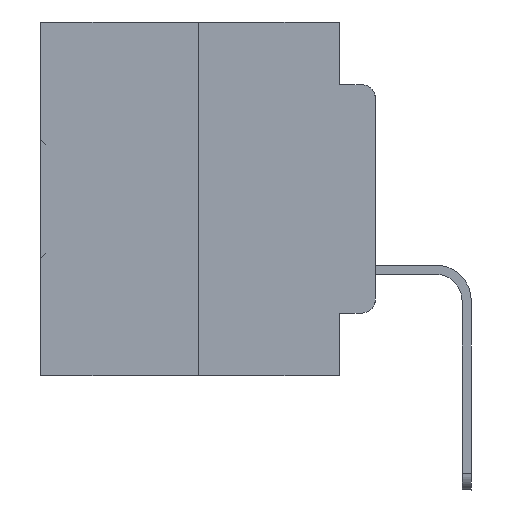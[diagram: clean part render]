
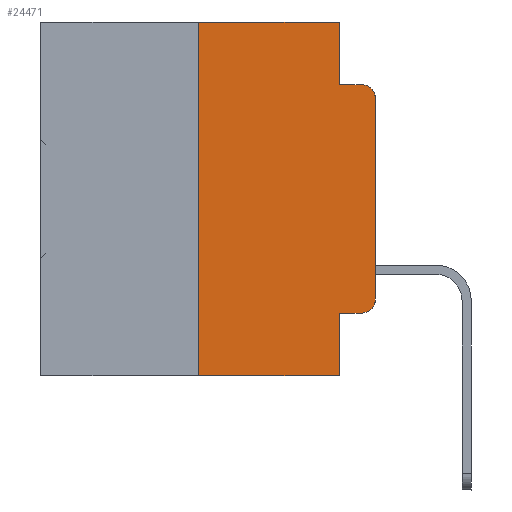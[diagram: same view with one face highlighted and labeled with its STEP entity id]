
A CAD part, left-side view. The second image highlights one B-rep face of the part: STEP entity #24471.
In plain terms, the highlighted planar face has unit normal (-1, 0, 0).
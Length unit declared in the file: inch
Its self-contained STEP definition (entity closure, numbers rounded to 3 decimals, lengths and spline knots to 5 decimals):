
#53 = EDGE_CURVE ( 'NONE', #14800, #1571, #8397, .T. ) ;
#319 = EDGE_CURVE ( 'NONE', #7575, #12504, #31278, .T. ) ;
#398 = CARTESIAN_POINT ( 'NONE',  ( 0., 0.473, 0. ) ) ;
#1571 = VERTEX_POINT ( 'NONE', #5385 ) ;
#2009 = VECTOR ( 'NONE', #22355, 39.37008 ) ;
#2048 = DIRECTION ( 'NONE',  ( 0., 0., 1. ) ) ;
#3149 = CARTESIAN_POINT ( 'NONE',  ( 0., 0.051, -0.0885 ) ) ;
#3265 = DIRECTION ( 'NONE',  ( 0., -1., 0. ) ) ;
#4979 = CARTESIAN_POINT ( 'NONE',  ( 0., 0.25, 0. ) ) ;
#5385 = CARTESIAN_POINT ( 'NONE',  ( 0., 0.02, -0.4115 ) ) ;
#5446 = DIRECTION ( 'NONE',  ( 0., 0., -1. ) ) ;
#5786 = CARTESIAN_POINT ( 'NONE',  ( 0., 0.473, 0. ) ) ;
#5818 = CIRCLE ( 'NONE', #23618, 0.02 ) ;
#5857 = CARTESIAN_POINT ( 'NONE',  ( 0., 0.051, 0. ) ) ;
#6010 = DIRECTION ( 'NONE',  ( 0., -1., 0. ) ) ;
#6371 = LINE ( 'NONE', #5786, #22662 ) ;
#6525 = EDGE_CURVE ( 'NONE', #14800, #15217, #8008, .T. ) ;
#6798 = CARTESIAN_POINT ( 'NONE',  ( 0., 0.02, -0.1085 ) ) ;
#6821 = CARTESIAN_POINT ( 'NONE',  ( 0., 0.051, -0.0885 ) ) ;
#6866 = EDGE_CURVE ( 'NONE', #22775, #15217, #16119, .T. ) ;
#7342 = EDGE_CURVE ( 'NONE', #12727, #27917, #7940, .T. ) ;
#7575 = VERTEX_POINT ( 'NONE', #9803 ) ;
#7852 = FACE_OUTER_BOUND ( 'NONE', #10377, .T. ) ;
#7940 = LINE ( 'NONE', #5857, #22614 ) ;
#8008 = LINE ( 'NONE', #22878, #21020 ) ;
#8397 = LINE ( 'NONE', #16643, #8834 ) ;
#8607 = VECTOR ( 'NONE', #32859, 39.37008 ) ;
#8613 = LINE ( 'NONE', #12088, #2009 ) ;
#8834 = VECTOR ( 'NONE', #20161, 39.37008 ) ;
#8839 = ORIENTED_EDGE ( 'NONE', *, *, #27946, .F. ) ;
#8915 = EDGE_CURVE ( 'NONE', #12504, #33897, #26978, .T. ) ;
#9507 = DIRECTION ( 'NONE',  ( 0., 0., -1. ) ) ;
#9710 = CARTESIAN_POINT ( 'NONE',  ( 0., 0.25, -0.5 ) ) ;
#9803 = CARTESIAN_POINT ( 'NONE',  ( 0., 0., -0.3915 ) ) ;
#10377 = EDGE_LOOP ( 'NONE', ( #31611, #15727, #30121, #11765, #8839, #25581, #11801, #24470, #13505, #22154 ) ) ;
#11185 = CARTESIAN_POINT ( 'NONE',  ( 0., 0.051, -0.4115 ) ) ;
#11765 = ORIENTED_EDGE ( 'NONE', *, *, #7342, .F. ) ;
#11801 = ORIENTED_EDGE ( 'NONE', *, *, #6866, .T. ) ;
#11934 = CARTESIAN_POINT ( 'NONE',  ( 0., 0.051, -0.5 ) ) ;
#11978 = AXIS2_PLACEMENT_3D ( 'NONE', #6798, #25012, #9507 ) ;
#12088 = CARTESIAN_POINT ( 'NONE',  ( 0., 0.25, 0. ) ) ;
#12365 = EDGE_CURVE ( 'NONE', #1571, #7575, #5818, .T. ) ;
#12504 = VERTEX_POINT ( 'NONE', #21328 ) ;
#12727 = VERTEX_POINT ( 'NONE', #30063 ) ;
#13059 = PLANE ( 'NONE',  #21486 ) ;
#13505 = ORIENTED_EDGE ( 'NONE', *, *, #53, .T. ) ;
#14800 = VERTEX_POINT ( 'NONE', #11185 ) ;
#14801 = DIRECTION ( 'NONE',  ( 0., 0., -1. ) ) ;
#15217 = VERTEX_POINT ( 'NONE', #11934 ) ;
#15727 = ORIENTED_EDGE ( 'NONE', *, *, #8915, .T. ) ;
#16119 = LINE ( 'NONE', #16453, #29641 ) ;
#16299 = DIRECTION ( 'NONE',  ( 0., 0., -1. ) ) ;
#16453 = CARTESIAN_POINT ( 'NONE',  ( 0., 0.473, -0.5 ) ) ;
#16643 = CARTESIAN_POINT ( 'NONE',  ( 0., 0.051, -0.4115 ) ) ;
#18079 = EDGE_CURVE ( 'NONE', #27917, #33897, #27358, .T. ) ;
#18781 = EDGE_CURVE ( 'NONE', #22775, #27675, #8613, .T. ) ;
#19354 = VECTOR ( 'NONE', #2048, 39.37008 ) ;
#20034 = CARTESIAN_POINT ( 'NONE',  ( 0., 0., 0. ) ) ;
#20161 = DIRECTION ( 'NONE',  ( 0., -1., 0. ) ) ;
#20626 = DIRECTION ( 'NONE',  ( -1., 0., 0. ) ) ;
#21020 = VECTOR ( 'NONE', #14801, 39.37008 ) ;
#21328 = CARTESIAN_POINT ( 'NONE',  ( 0., 0., -0.1085 ) ) ;
#21486 = AXIS2_PLACEMENT_3D ( 'NONE', #398, #29082, #5446 ) ;
#22154 = ORIENTED_EDGE ( 'NONE', *, *, #12365, .T. ) ;
#22355 = DIRECTION ( 'NONE',  ( 0., 0., 1. ) ) ;
#22614 = VECTOR ( 'NONE', #16299, 39.37008 ) ;
#22662 = VECTOR ( 'NONE', #3265, 39.37008 ) ;
#22775 = VERTEX_POINT ( 'NONE', #9710 ) ;
#22878 = CARTESIAN_POINT ( 'NONE',  ( 0., 0.051, 0. ) ) ;
#23381 = DIRECTION ( 'NONE',  ( 0., 0., -1. ) ) ;
#23618 = AXIS2_PLACEMENT_3D ( 'NONE', #26012, #20626, #23381 ) ;
#24470 = ORIENTED_EDGE ( 'NONE', *, *, #6525, .F. ) ;
#24471 = ADVANCED_FACE ( 'NONE', ( #7852 ), #13059, .F. ) ;
#25012 = DIRECTION ( 'NONE',  ( -1., 0., 0. ) ) ;
#25581 = ORIENTED_EDGE ( 'NONE', *, *, #18781, .F. ) ;
#26012 = CARTESIAN_POINT ( 'NONE',  ( 0., 0.02, -0.3915 ) ) ;
#26978 = CIRCLE ( 'NONE', #11978, 0.02 ) ;
#27358 = LINE ( 'NONE', #6821, #8607 ) ;
#27675 = VERTEX_POINT ( 'NONE', #4979 ) ;
#27917 = VERTEX_POINT ( 'NONE', #3149 ) ;
#27946 = EDGE_CURVE ( 'NONE', #27675, #12727, #6371, .T. ) ;
#29082 = DIRECTION ( 'NONE',  ( 1., 0., 0. ) ) ;
#29641 = VECTOR ( 'NONE', #6010, 39.37008 ) ;
#30063 = CARTESIAN_POINT ( 'NONE',  ( 0., 0.051, 0. ) ) ;
#30121 = ORIENTED_EDGE ( 'NONE', *, *, #18079, .F. ) ;
#30928 = CARTESIAN_POINT ( 'NONE',  ( 0., 0.02, -0.0885 ) ) ;
#31278 = LINE ( 'NONE', #20034, #19354 ) ;
#31611 = ORIENTED_EDGE ( 'NONE', *, *, #319, .T. ) ;
#32859 = DIRECTION ( 'NONE',  ( 0., -1., 0. ) ) ;
#33897 = VERTEX_POINT ( 'NONE', #30928 ) ;
